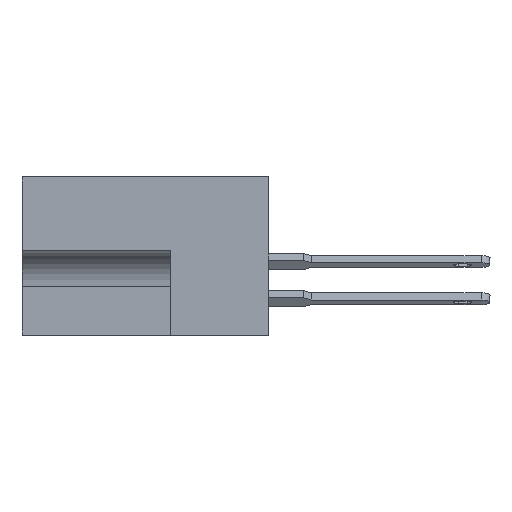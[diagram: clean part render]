
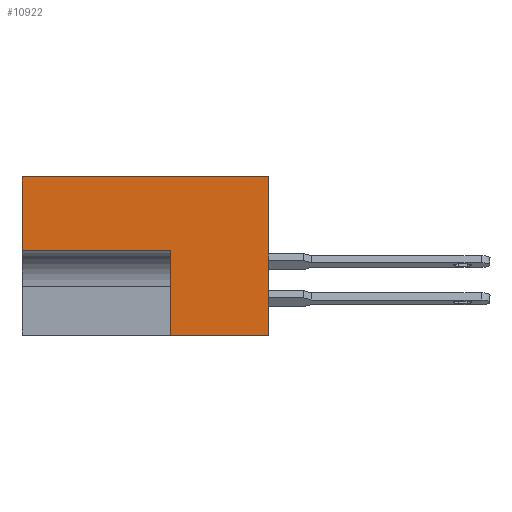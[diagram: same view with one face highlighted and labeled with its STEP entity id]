
A CAD part, left-side view. The second image highlights one B-rep face of the part: STEP entity #10922.
In plain terms, the highlighted planar face has unit normal (-1, 0, 0).
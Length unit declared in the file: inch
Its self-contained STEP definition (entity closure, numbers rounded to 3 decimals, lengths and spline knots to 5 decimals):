
#436 = EDGE_CURVE ( 'NONE', #11884, #9381, #5052, .T. ) ;
#718 = DIRECTION ( 'NONE',  ( 0., -1., 0. ) ) ;
#1729 = LINE ( 'NONE', #14886, #14947 ) ;
#1756 = EDGE_LOOP ( 'NONE', ( #19320, #14569, #16875, #5167, #13917, #17149 ) ) ;
#1863 = DIRECTION ( 'NONE',  ( 0., 0., 1. ) ) ;
#2048 = CARTESIAN_POINT ( 'NONE',  ( 0., 0., -0.531 ) ) ;
#2075 = DIRECTION ( 'NONE',  ( 0., 0., 1. ) ) ;
#3024 = VECTOR ( 'NONE', #12329, 39.37008 ) ;
#3346 = VECTOR ( 'NONE', #2075, 39.37008 ) ;
#3680 = CARTESIAN_POINT ( 'NONE',  ( 0., 0.453, 0. ) ) ;
#4047 = LINE ( 'NONE', #11557, #3346 ) ;
#4665 = LINE ( 'NONE', #14080, #13790 ) ;
#5052 = LINE ( 'NONE', #12995, #6481 ) ;
#5167 = ORIENTED_EDGE ( 'NONE', *, *, #18034, .T. ) ;
#5251 = AXIS2_PLACEMENT_3D ( 'NONE', #3680, #11628, #14360 ) ;
#5691 = DIRECTION ( 'NONE',  ( 0., -1., 0. ) ) ;
#6481 = VECTOR ( 'NONE', #13130, 39.37008 ) ;
#6634 = CARTESIAN_POINT ( 'NONE',  ( 0., 0.828, -0.248 ) ) ;
#6744 = CARTESIAN_POINT ( 'NONE',  ( 0., 0.328, -0.531 ) ) ;
#8197 = LINE ( 'NONE', #8362, #18977 ) ;
#8362 = CARTESIAN_POINT ( 'NONE',  ( 0., 0.453, 0. ) ) ;
#8656 = EDGE_CURVE ( 'NONE', #18466, #19769, #4665, .T. ) ;
#8678 = VERTEX_POINT ( 'NONE', #2048 ) ;
#9381 = VERTEX_POINT ( 'NONE', #17778 ) ;
#10922 = ADVANCED_FACE ( 'NONE', ( #13438 ), #11372, .F. ) ;
#11372 = PLANE ( 'NONE',  #5251 ) ;
#11557 = CARTESIAN_POINT ( 'NONE',  ( 0., 0., 0. ) ) ;
#11628 = DIRECTION ( 'NONE',  ( 1., 0., 0. ) ) ;
#11884 = VERTEX_POINT ( 'NONE', #6634 ) ;
#12329 = DIRECTION ( 'NONE',  ( 0., 1., 0. ) ) ;
#12995 = CARTESIAN_POINT ( 'NONE',  ( 0., 0.828, 0. ) ) ;
#13130 = DIRECTION ( 'NONE',  ( 0., 0., 1. ) ) ;
#13438 = FACE_OUTER_BOUND ( 'NONE', #1756, .T. ) ;
#13780 = CARTESIAN_POINT ( 'NONE',  ( 0., 0.328, -0.248 ) ) ;
#13790 = VECTOR ( 'NONE', #1863, 39.37008 ) ;
#13917 = ORIENTED_EDGE ( 'NONE', *, *, #19747, .T. ) ;
#14080 = CARTESIAN_POINT ( 'NONE',  ( 0., 0.328, -0.531 ) ) ;
#14097 = VERTEX_POINT ( 'NONE', #16662 ) ;
#14360 = DIRECTION ( 'NONE',  ( 0., 0., -1. ) ) ;
#14569 = ORIENTED_EDGE ( 'NONE', *, *, #16195, .F. ) ;
#14886 = CARTESIAN_POINT ( 'NONE',  ( 0., 0.453, -0.531 ) ) ;
#14947 = VECTOR ( 'NONE', #5691, 39.37008 ) ;
#16195 = EDGE_CURVE ( 'NONE', #19769, #11884, #19090, .T. ) ;
#16662 = CARTESIAN_POINT ( 'NONE',  ( 0., 0., 0. ) ) ;
#16875 = ORIENTED_EDGE ( 'NONE', *, *, #8656, .F. ) ;
#17149 = ORIENTED_EDGE ( 'NONE', *, *, #18535, .F. ) ;
#17616 = CARTESIAN_POINT ( 'NONE',  ( 0., 0.328, -0.248 ) ) ;
#17778 = CARTESIAN_POINT ( 'NONE',  ( 0., 0.828, 0. ) ) ;
#18034 = EDGE_CURVE ( 'NONE', #18466, #8678, #1729, .T. ) ;
#18466 = VERTEX_POINT ( 'NONE', #6744 ) ;
#18535 = EDGE_CURVE ( 'NONE', #9381, #14097, #8197, .T. ) ;
#18977 = VECTOR ( 'NONE', #718, 39.37008 ) ;
#19090 = LINE ( 'NONE', #13780, #3024 ) ;
#19320 = ORIENTED_EDGE ( 'NONE', *, *, #436, .F. ) ;
#19747 = EDGE_CURVE ( 'NONE', #8678, #14097, #4047, .T. ) ;
#19769 = VERTEX_POINT ( 'NONE', #17616 ) ;
